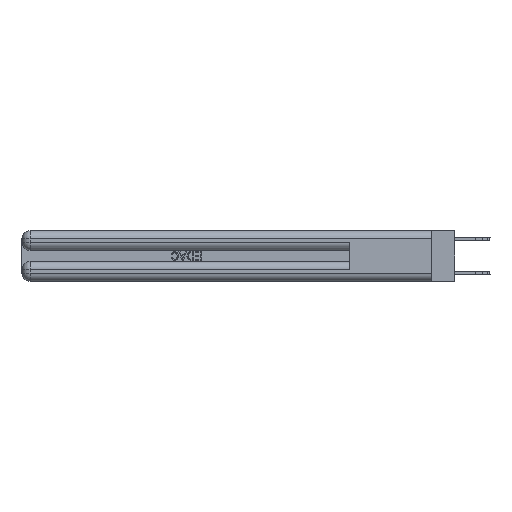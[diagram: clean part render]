
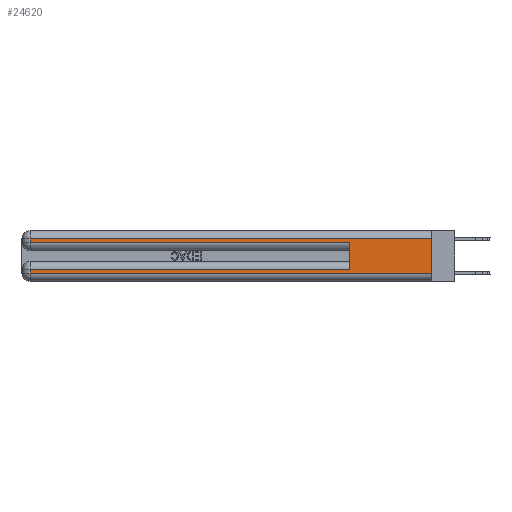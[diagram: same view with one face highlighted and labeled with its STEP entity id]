
A CAD part, left-side view. The second image highlights one B-rep face of the part: STEP entity #24620.
In plain terms, the highlighted planar face has unit normal (-1, 0, 0).
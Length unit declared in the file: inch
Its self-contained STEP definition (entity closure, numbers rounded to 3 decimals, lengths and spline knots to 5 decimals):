
#248 = LINE ( 'NONE', #9364, #3070 ) ;
#414 = LINE ( 'NONE', #18923, #10820 ) ;
#588 = CARTESIAN_POINT ( 'NONE',  ( 0., 2.94, 0.285 ) ) ;
#887 = EDGE_CURVE ( 'NONE', #7053, #20914, #248, .T. ) ;
#962 = CARTESIAN_POINT ( 'NONE',  ( 0., 0.6, 0.145 ) ) ;
#1524 = FACE_OUTER_BOUND ( 'NONE', #17478, .T. ) ;
#2350 = CARTESIAN_POINT ( 'NONE',  ( 0., 2.94, 0.06 ) ) ;
#2375 = ORIENTED_EDGE ( 'NONE', *, *, #7051, .F. ) ;
#2735 = CARTESIAN_POINT ( 'NONE',  ( 0., 2.94, 0.31 ) ) ;
#2906 = EDGE_CURVE ( 'NONE', #10713, #7053, #6333, .T. ) ;
#2922 = DIRECTION ( 'NONE',  ( 0., 0., -1. ) ) ;
#2996 = CARTESIAN_POINT ( 'NONE',  ( 0., 0., 0.37 ) ) ;
#3070 = VECTOR ( 'NONE', #2922, 39.37008 ) ;
#3324 = DIRECTION ( 'NONE',  ( 0., 0., -1. ) ) ;
#3483 = VECTOR ( 'NONE', #10066, 39.37008 ) ;
#4387 = ORIENTED_EDGE ( 'NONE', *, *, #12007, .T. ) ;
#4551 = CARTESIAN_POINT ( 'NONE',  ( 0., 0., 0.31 ) ) ;
#6285 = ORIENTED_EDGE ( 'NONE', *, *, #2906, .T. ) ;
#6333 = LINE ( 'NONE', #27063, #27212 ) ;
#6666 = VECTOR ( 'NONE', #9869, 39.37008 ) ;
#6725 = VERTEX_POINT ( 'NONE', #588 ) ;
#7051 = EDGE_CURVE ( 'NONE', #10713, #8109, #12147, .T. ) ;
#7053 = VERTEX_POINT ( 'NONE', #21565 ) ;
#7593 = EDGE_CURVE ( 'NONE', #26308, #6725, #17956, .T. ) ;
#7775 = LINE ( 'NONE', #2996, #6666 ) ;
#8109 = VERTEX_POINT ( 'NONE', #22081 ) ;
#9364 = CARTESIAN_POINT ( 'NONE',  ( 0., 2.94, 0.37 ) ) ;
#9514 = VERTEX_POINT ( 'NONE', #4551 ) ;
#9532 = DIRECTION ( 'NONE',  ( 0., -1., 0. ) ) ;
#9869 = DIRECTION ( 'NONE',  ( 0., 0., -1. ) ) ;
#10051 = ORIENTED_EDGE ( 'NONE', *, *, #19541, .T. ) ;
#10066 = DIRECTION ( 'NONE',  ( 0., 0., 1. ) ) ;
#10713 = VERTEX_POINT ( 'NONE', #16259 ) ;
#10820 = VECTOR ( 'NONE', #9532, 39.37008 ) ;
#10889 = ORIENTED_EDGE ( 'NONE', *, *, #25568, .T. ) ;
#11088 = VERTEX_POINT ( 'NONE', #26952 ) ;
#11555 = ORIENTED_EDGE ( 'NONE', *, *, #7593, .T. ) ;
#12007 = EDGE_CURVE ( 'NONE', #20914, #11088, #414, .T. ) ;
#12147 = LINE ( 'NONE', #962, #3483 ) ;
#12918 = ORIENTED_EDGE ( 'NONE', *, *, #14333, .F. ) ;
#13173 = DIRECTION ( 'NONE',  ( 0., 1., 0. ) ) ;
#13516 = CARTESIAN_POINT ( 'NONE',  ( 0., 0., 0.31 ) ) ;
#13524 = VECTOR ( 'NONE', #16592, 39.37008 ) ;
#14333 = EDGE_CURVE ( 'NONE', #9514, #11088, #7775, .T. ) ;
#16259 = CARTESIAN_POINT ( 'NONE',  ( 0., 0.6, 0.085 ) ) ;
#16592 = DIRECTION ( 'NONE',  ( 0., -1., 0. ) ) ;
#16924 = CARTESIAN_POINT ( 'NONE',  ( 0., 0., 0.37 ) ) ;
#17080 = DIRECTION ( 'NONE',  ( 1., 0., 0. ) ) ;
#17364 = DIRECTION ( 'NONE',  ( 0., 0., -1. ) ) ;
#17478 = EDGE_LOOP ( 'NONE', ( #12918, #10051, #11555, #10889, #2375, #6285, #27156, #4387 ) ) ;
#17956 = LINE ( 'NONE', #27031, #29133 ) ;
#18923 = CARTESIAN_POINT ( 'NONE',  ( 0., 0., 0.06 ) ) ;
#19541 = EDGE_CURVE ( 'NONE', #9514, #26308, #25020, .T. ) ;
#20914 = VERTEX_POINT ( 'NONE', #2350 ) ;
#21565 = CARTESIAN_POINT ( 'NONE',  ( 0., 2.94, 0.085 ) ) ;
#22081 = CARTESIAN_POINT ( 'NONE',  ( 0., 0.6, 0.285 ) ) ;
#22678 = AXIS2_PLACEMENT_3D ( 'NONE', #16924, #17080, #3324 ) ;
#22988 = VECTOR ( 'NONE', #24577, 39.37008 ) ;
#24577 = DIRECTION ( 'NONE',  ( 0., 1., 0. ) ) ;
#24620 = ADVANCED_FACE ( 'NONE', ( #1524 ), #26160, .F. ) ;
#25020 = LINE ( 'NONE', #13516, #22988 ) ;
#25568 = EDGE_CURVE ( 'NONE', #6725, #8109, #25684, .T. ) ;
#25684 = LINE ( 'NONE', #27766, #13524 ) ;
#26160 = PLANE ( 'NONE',  #22678 ) ;
#26308 = VERTEX_POINT ( 'NONE', #2735 ) ;
#26952 = CARTESIAN_POINT ( 'NONE',  ( 0., 0., 0.06 ) ) ;
#27031 = CARTESIAN_POINT ( 'NONE',  ( 0., 2.94, 0.37 ) ) ;
#27063 = CARTESIAN_POINT ( 'NONE',  ( 0., 0., 0.085 ) ) ;
#27156 = ORIENTED_EDGE ( 'NONE', *, *, #887, .T. ) ;
#27212 = VECTOR ( 'NONE', #13173, 39.37008 ) ;
#27766 = CARTESIAN_POINT ( 'NONE',  ( 0., 0., 0.285 ) ) ;
#29133 = VECTOR ( 'NONE', #17364, 39.37008 ) ;
